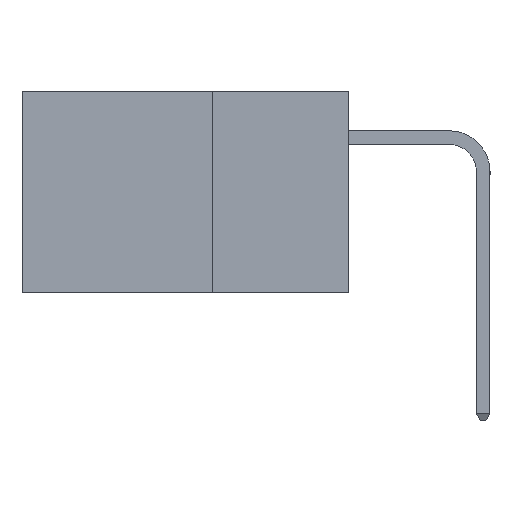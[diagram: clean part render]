
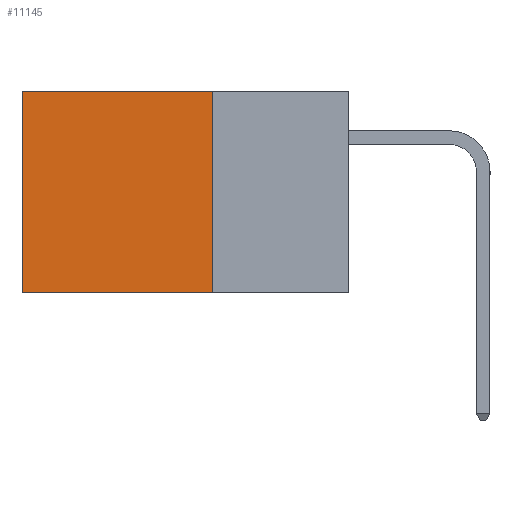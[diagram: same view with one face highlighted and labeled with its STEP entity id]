
A CAD part, left-side view. The second image highlights one B-rep face of the part: STEP entity #11145.
In plain terms, the highlighted planar face has unit normal (-1, 0, 0).
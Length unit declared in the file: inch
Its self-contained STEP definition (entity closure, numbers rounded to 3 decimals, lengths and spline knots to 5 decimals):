
#852 = ORIENTED_EDGE ( 'NONE', *, *, #8689, .F. ) ;
#1503 = CARTESIAN_POINT ( 'NONE',  ( 0.2875, 0.6, -0.37 ) ) ;
#1757 = LINE ( 'NONE', #8181, #11626 ) ;
#2208 = VERTEX_POINT ( 'NONE', #1503 ) ;
#2923 = CARTESIAN_POINT ( 'NONE',  ( 0.2875, 0.25, 0. ) ) ;
#3330 = CARTESIAN_POINT ( 'NONE',  ( 0.2875, 0.6, 0. ) ) ;
#3500 = EDGE_CURVE ( 'NONE', #10149, #2208, #4818, .T. ) ;
#3563 = LINE ( 'NONE', #8411, #5765 ) ;
#4240 = FACE_OUTER_BOUND ( 'NONE', #8942, .T. ) ;
#4334 = DIRECTION ( 'NONE',  ( 0., 0., -1. ) ) ;
#4666 = ORIENTED_EDGE ( 'NONE', *, *, #6875, .F. ) ;
#4818 = LINE ( 'NONE', #9828, #12402 ) ;
#5274 = VECTOR ( 'NONE', #10045, 39.37008 ) ;
#5377 = DIRECTION ( 'NONE',  ( 0., 0., -1. ) ) ;
#5765 = VECTOR ( 'NONE', #7450, 39.37008 ) ;
#6081 = VERTEX_POINT ( 'NONE', #6896 ) ;
#6702 = DIRECTION ( 'NONE',  ( 0., 0., -1. ) ) ;
#6875 = EDGE_CURVE ( 'NONE', #6081, #2208, #8081, .T. ) ;
#6896 = CARTESIAN_POINT ( 'NONE',  ( 0.2875, 0.25, -0.37 ) ) ;
#7450 = DIRECTION ( 'NONE',  ( 0., 1., 0. ) ) ;
#8081 = LINE ( 'NONE', #10986, #5274 ) ;
#8181 = CARTESIAN_POINT ( 'NONE',  ( 0.2875, 0.25, 0. ) ) ;
#8411 = CARTESIAN_POINT ( 'NONE',  ( 0.2875, 0.25, 0. ) ) ;
#8478 = ORIENTED_EDGE ( 'NONE', *, *, #9854, .T. ) ;
#8625 = AXIS2_PLACEMENT_3D ( 'NONE', #2923, #12459, #6702 ) ;
#8689 = EDGE_CURVE ( 'NONE', #9810, #6081, #1757, .T. ) ;
#8942 = EDGE_LOOP ( 'NONE', ( #9522, #4666, #852, #8478 ) ) ;
#9314 = CARTESIAN_POINT ( 'NONE',  ( 0.2875, 0.25, 0. ) ) ;
#9522 = ORIENTED_EDGE ( 'NONE', *, *, #3500, .T. ) ;
#9810 = VERTEX_POINT ( 'NONE', #9314 ) ;
#9828 = CARTESIAN_POINT ( 'NONE',  ( 0.2875, 0.6, 0. ) ) ;
#9854 = EDGE_CURVE ( 'NONE', #9810, #10149, #3563, .T. ) ;
#10045 = DIRECTION ( 'NONE',  ( 0., 1., 0. ) ) ;
#10149 = VERTEX_POINT ( 'NONE', #3330 ) ;
#10512 = PLANE ( 'NONE',  #8625 ) ;
#10986 = CARTESIAN_POINT ( 'NONE',  ( 0.2875, 0.25, -0.37 ) ) ;
#11145 = ADVANCED_FACE ( 'NONE', ( #4240 ), #10512, .F. ) ;
#11626 = VECTOR ( 'NONE', #5377, 39.37008 ) ;
#12402 = VECTOR ( 'NONE', #4334, 39.37008 ) ;
#12459 = DIRECTION ( 'NONE',  ( 1., 0., 0. ) ) ;
